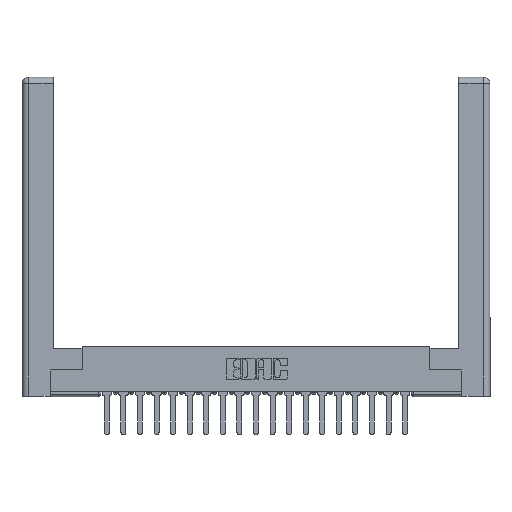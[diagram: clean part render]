
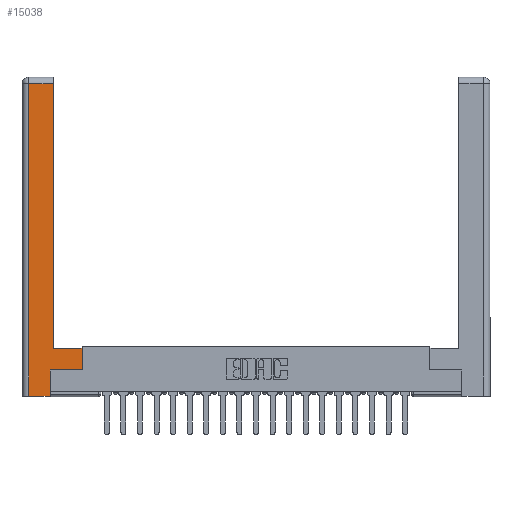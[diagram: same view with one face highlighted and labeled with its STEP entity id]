
A CAD part, top view. The second image highlights one B-rep face of the part: STEP entity #15038.
In plain terms, the highlighted planar face has unit normal (0, 0, 1).
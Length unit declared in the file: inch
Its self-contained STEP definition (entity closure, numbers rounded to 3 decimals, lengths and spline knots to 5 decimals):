
#271 = VECTOR ( 'NONE', #1358, 39.37008 ) ;
#410 = LINE ( 'NONE', #20779, #17721 ) ;
#500 = VECTOR ( 'NONE', #16580, 39.37008 ) ;
#655 = ORIENTED_EDGE ( 'NONE', *, *, #2217, .T. ) ;
#1043 = CARTESIAN_POINT ( 'NONE',  ( 0.565, 0.45, 0. ) ) ;
#1358 = DIRECTION ( 'NONE',  ( 1., 0., 0. ) ) ;
#2217 = EDGE_CURVE ( 'NONE', #16183, #19338, #8665, .T. ) ;
#2339 = DIRECTION ( 'NONE',  ( -1., 0., 0. ) ) ;
#2646 = CARTESIAN_POINT ( 'NONE',  ( 0.565, 0.245, 0. ) ) ;
#2832 = ORIENTED_EDGE ( 'NONE', *, *, #12616, .T. ) ;
#3088 = EDGE_CURVE ( 'NONE', #11120, #10389, #17256, .T. ) ;
#3404 = ORIENTED_EDGE ( 'NONE', *, *, #15086, .T. ) ;
#3475 = DIRECTION ( 'NONE',  ( 0., 1., 0. ) ) ;
#3999 = VECTOR ( 'NONE', #14731, 39.37008 ) ;
#4387 = VECTOR ( 'NONE', #20091, 39.37008 ) ;
#4473 = LINE ( 'NONE', #1043, #9973 ) ;
#4685 = DIRECTION ( 'NONE',  ( 0., 0., -1. ) ) ;
#4735 = VECTOR ( 'NONE', #17436, 39.37008 ) ;
#4740 = CARTESIAN_POINT ( 'NONE',  ( 0.295, 0.45, 0. ) ) ;
#5390 = CARTESIAN_POINT ( 'NONE',  ( 0.295, 2.94, 0. ) ) ;
#5433 = VERTEX_POINT ( 'NONE', #12489 ) ;
#6296 = DIRECTION ( 'NONE',  ( -1., 0., 0. ) ) ;
#6311 = VERTEX_POINT ( 'NONE', #12034 ) ;
#6558 = LINE ( 'NONE', #21632, #500 ) ;
#6795 = CARTESIAN_POINT ( 'NONE',  ( 0.0615, 2.94, 0. ) ) ;
#7579 = ORIENTED_EDGE ( 'NONE', *, *, #20615, .T. ) ;
#8049 = PLANE ( 'NONE',  #13065 ) ;
#8285 = ORIENTED_EDGE ( 'NONE', *, *, #15788, .T. ) ;
#8606 = CARTESIAN_POINT ( 'NONE',  ( 0.295, 3., 0. ) ) ;
#8665 = LINE ( 'NONE', #2646, #4735 ) ;
#8708 = LINE ( 'NONE', #11356, #3999 ) ;
#9057 = EDGE_CURVE ( 'NONE', #19338, #6311, #4473, .T. ) ;
#9973 = VECTOR ( 'NONE', #16086, 39.37008 ) ;
#10389 = VERTEX_POINT ( 'NONE', #5390 ) ;
#11120 = VERTEX_POINT ( 'NONE', #4740 ) ;
#11356 = CARTESIAN_POINT ( 'NONE',  ( 0.0615, 0., 0. ) ) ;
#11422 = CARTESIAN_POINT ( 'NONE',  ( 0., 0., 0. ) ) ;
#12034 = CARTESIAN_POINT ( 'NONE',  ( 0.565, 0.45, 0. ) ) ;
#12276 = VECTOR ( 'NONE', #3475, 39.37008 ) ;
#12320 = ORIENTED_EDGE ( 'NONE', *, *, #9057, .T. ) ;
#12435 = VERTEX_POINT ( 'NONE', #15307 ) ;
#12489 = CARTESIAN_POINT ( 'NONE',  ( 0.0615, 0., 0. ) ) ;
#12616 = EDGE_CURVE ( 'NONE', #10389, #20216, #410, .T. ) ;
#13065 = AXIS2_PLACEMENT_3D ( 'NONE', #11422, #4685, #6296 ) ;
#13151 = LINE ( 'NONE', #19744, #271 ) ;
#13802 = CARTESIAN_POINT ( 'NONE',  ( 0.565, 0.245, 0. ) ) ;
#14731 = DIRECTION ( 'NONE',  ( 0., -1., 0. ) ) ;
#15038 = ADVANCED_FACE ( 'NONE', ( #19712 ), #8049, .F. ) ;
#15086 = EDGE_CURVE ( 'NONE', #20216, #5433, #8708, .T. ) ;
#15307 = CARTESIAN_POINT ( 'NONE',  ( 0.265, 0., 0. ) ) ;
#15788 = EDGE_CURVE ( 'NONE', #6311, #11120, #6558, .T. ) ;
#16086 = DIRECTION ( 'NONE',  ( 0., 1., 0. ) ) ;
#16183 = VERTEX_POINT ( 'NONE', #19263 ) ;
#16254 = ORIENTED_EDGE ( 'NONE', *, *, #17335, .T. ) ;
#16580 = DIRECTION ( 'NONE',  ( -1., 0., 0. ) ) ;
#16852 = ORIENTED_EDGE ( 'NONE', *, *, #3088, .T. ) ;
#17256 = LINE ( 'NONE', #8606, #12276 ) ;
#17335 = EDGE_CURVE ( 'NONE', #12435, #16183, #19045, .T. ) ;
#17436 = DIRECTION ( 'NONE',  ( 1., 0., 0. ) ) ;
#17721 = VECTOR ( 'NONE', #2339, 39.37008 ) ;
#18240 = CARTESIAN_POINT ( 'NONE',  ( 0.265, 0.245, 0. ) ) ;
#18513 = EDGE_LOOP ( 'NONE', ( #16852, #2832, #3404, #7579, #16254, #655, #12320, #8285 ) ) ;
#19045 = LINE ( 'NONE', #18240, #4387 ) ;
#19263 = CARTESIAN_POINT ( 'NONE',  ( 0.265, 0.245, 0. ) ) ;
#19338 = VERTEX_POINT ( 'NONE', #13802 ) ;
#19712 = FACE_OUTER_BOUND ( 'NONE', #18513, .T. ) ;
#19744 = CARTESIAN_POINT ( 'NONE',  ( 0.265, 0., 0. ) ) ;
#20091 = DIRECTION ( 'NONE',  ( 0., 1., 0. ) ) ;
#20216 = VERTEX_POINT ( 'NONE', #6795 ) ;
#20615 = EDGE_CURVE ( 'NONE', #5433, #12435, #13151, .T. ) ;
#20779 = CARTESIAN_POINT ( 'NONE',  ( 0.0615, 2.94, 0. ) ) ;
#21632 = CARTESIAN_POINT ( 'NONE',  ( 0.295, 0.45, 0. ) ) ;
